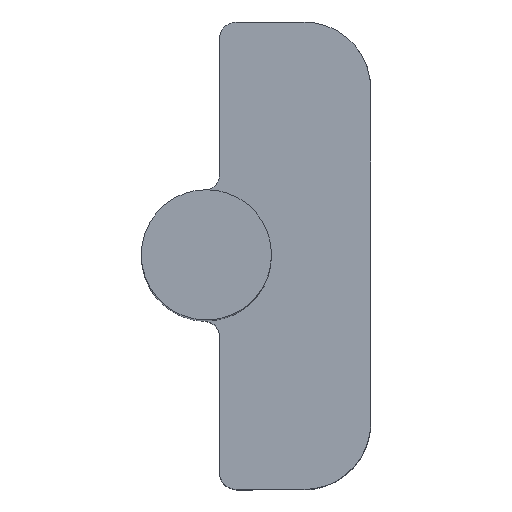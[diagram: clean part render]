
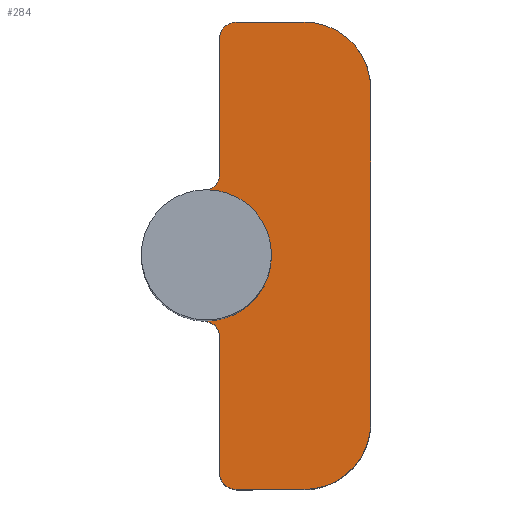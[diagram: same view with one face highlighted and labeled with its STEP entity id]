
A CAD part, top view. The second image highlights one B-rep face of the part: STEP entity #284.
In plain terms, the highlighted planar face has unit normal (0, 0, 1).
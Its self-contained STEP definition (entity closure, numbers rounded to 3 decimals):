
#15=CIRCLE('',#307,2.);
#21=CIRCLE('',#315,0.5);
#22=CIRCLE('',#318,0.5);
#24=CIRCLE('',#321,1.95);
#25=CIRCLE('',#322,1.95);
#26=CIRCLE('',#324,0.5);
#27=CIRCLE('',#327,0.5);
#28=CIRCLE('',#330,2.);
#47=FACE_OUTER_BOUND('',#63,.T.);
#63=EDGE_LOOP('',(#238,#239,#240,#241,#242,#243,#244,#245,#246,#247,#248,
#249,#250));
#79=LINE('',#468,#103);
#86=LINE('',#491,#110);
#88=LINE('',#497,#112);
#89=LINE('',#501,#113);
#90=LINE('',#502,#114);
#103=VECTOR('',#376,10.);
#110=VECTOR('',#401,10.);
#112=VECTOR('',#409,10.);
#113=VECTOR('',#414,10.);
#114=VECTOR('',#415,10.);
#122=VERTEX_POINT('',#436);
#123=VERTEX_POINT('',#438);
#132=VERTEX_POINT('',#460);
#133=VERTEX_POINT('',#461);
#134=VERTEX_POINT('',#466);
#135=VERTEX_POINT('',#470);
#136=VERTEX_POINT('',#471);
#138=VERTEX_POINT('',#478);
#139=VERTEX_POINT('',#480);
#140=VERTEX_POINT('',#485);
#141=VERTEX_POINT('',#486);
#142=VERTEX_POINT('',#493);
#143=VERTEX_POINT('',#499);
#149=EDGE_CURVE('',#122,#123,#15,.T.);
#160=EDGE_CURVE('',#132,#133,#21,.T.);
#164=EDGE_CURVE('',#134,#132,#79,.T.);
#165=EDGE_CURVE('',#135,#136,#22,.T.);
#170=EDGE_CURVE('',#139,#138,#24,.T.);
#172=EDGE_CURVE('',#138,#136,#25,.T.);
#173=EDGE_CURVE('',#140,#141,#26,.T.);
#176=EDGE_CURVE('',#141,#122,#86,.F.);
#177=EDGE_CURVE('',#139,#142,#27,.T.);
#179=EDGE_CURVE('',#140,#142,#88,.F.);
#180=EDGE_CURVE('',#143,#134,#28,.T.);
#181=EDGE_CURVE('',#123,#143,#89,.T.);
#182=EDGE_CURVE('',#135,#133,#90,.F.);
#238=ORIENTED_EDGE('',*,*,#160,.F.);
#239=ORIENTED_EDGE('',*,*,#164,.F.);
#240=ORIENTED_EDGE('',*,*,#180,.F.);
#241=ORIENTED_EDGE('',*,*,#181,.F.);
#242=ORIENTED_EDGE('',*,*,#149,.F.);
#243=ORIENTED_EDGE('',*,*,#176,.F.);
#244=ORIENTED_EDGE('',*,*,#173,.F.);
#245=ORIENTED_EDGE('',*,*,#179,.T.);
#246=ORIENTED_EDGE('',*,*,#177,.F.);
#247=ORIENTED_EDGE('',*,*,#170,.T.);
#248=ORIENTED_EDGE('',*,*,#172,.T.);
#249=ORIENTED_EDGE('',*,*,#165,.F.);
#250=ORIENTED_EDGE('',*,*,#182,.T.);
#269=PLANE('',#329);
#284=ADVANCED_FACE('',(#47),#269,.F.);
#307=AXIS2_PLACEMENT_3D('',#439,#348,#349);
#315=AXIS2_PLACEMENT_3D('',#462,#369,#370);
#318=AXIS2_PLACEMENT_3D('',#472,#379,#380);
#321=AXIS2_PLACEMENT_3D('',#481,#388,#389);
#322=AXIS2_PLACEMENT_3D('',#483,#391,#392);
#324=AXIS2_PLACEMENT_3D('',#487,#395,#396);
#327=AXIS2_PLACEMENT_3D('',#494,#404,#405);
#329=AXIS2_PLACEMENT_3D('',#498,#410,#411);
#330=AXIS2_PLACEMENT_3D('',#500,#412,#413);
#348=DIRECTION('center_axis',(0.,0.,
-1.));
#349=DIRECTION('ref_axis',(0.707,0.707,0.));
#369=DIRECTION('center_axis',(0.,0.,
-1.));
#370=DIRECTION('ref_axis',(-0.707,-0.707,0.));
#376=DIRECTION('',(-1.,0.,0.));
#379=DIRECTION('center_axis',(0.,0.,
1.));
#380=DIRECTION('ref_axis',(0.721,0.693,0.));
#388=DIRECTION('center_axis',(0.,0.,
-1.));
#389=DIRECTION('ref_axis',(-1.,0.,0.));
#391=DIRECTION('center_axis',(0.,0.,
-1.));
#392=DIRECTION('ref_axis',(-1.,0.,0.));
#395=DIRECTION('center_axis',(0.,0.,
-1.));
#396=DIRECTION('ref_axis',(-0.707,0.707,0.));
#401=DIRECTION('',(-1.,0.,0.));
#404=DIRECTION('center_axis',(0.,0.,
1.));
#405=DIRECTION('ref_axis',(0.721,-0.693,0.));
#409=DIRECTION('',(0.,1.,0.));
#410=DIRECTION('center_axis',(0.,0.,
-1.));
#411=DIRECTION('ref_axis',(0.,1.,0.));
#412=DIRECTION('center_axis',(0.,0.,
-1.));
#413=DIRECTION('ref_axis',(0.707,-0.707,0.));
#414=DIRECTION('',(0.,-1.,0.));
#415=DIRECTION('',(0.,1.,0.));
#436=CARTESIAN_POINT('',(2.922,7.,32.8));
#438=CARTESIAN_POINT('',(4.922,5.,32.8));
#439=CARTESIAN_POINT('Origin',(2.922,5.,32.8));
#460=CARTESIAN_POINT('',(0.9,-7.,32.8));
#461=CARTESIAN_POINT('',(0.4,-6.5,32.8));
#462=CARTESIAN_POINT('Origin',(0.9,-6.5,32.8));
#466=CARTESIAN_POINT('',(2.922,-7.,32.8));
#468=CARTESIAN_POINT('',(2.5,-7.,32.8));
#470=CARTESIAN_POINT('',(0.4,-2.448,32.8));
#471=CARTESIAN_POINT('',(-0.08,-1.948,32.8));
#472=CARTESIAN_POINT('Origin',(-0.1,-2.448,32.8));
#478=CARTESIAN_POINT('',(1.95,0.,32.8));
#480=CARTESIAN_POINT('',(-0.08,1.948,32.8));
#481=CARTESIAN_POINT('Origin',(0.,0.,
32.8));
#483=CARTESIAN_POINT('Origin',(0.,0.,
32.8));
#485=CARTESIAN_POINT('',(0.4,6.5,32.8));
#486=CARTESIAN_POINT('',(0.9,7.,32.8));
#487=CARTESIAN_POINT('Origin',(0.9,6.5,32.8));
#491=CARTESIAN_POINT('',(2.5,7.,32.8));
#493=CARTESIAN_POINT('',(0.4,2.448,32.8));
#494=CARTESIAN_POINT('Origin',(-0.1,2.448,32.8));
#497=CARTESIAN_POINT('',(0.4,3.45,32.8));
#498=CARTESIAN_POINT('Origin',(2.5,3.45,32.8));
#499=CARTESIAN_POINT('',(4.922,-5.,32.8));
#500=CARTESIAN_POINT('Origin',(2.922,-5.,32.8));
#501=CARTESIAN_POINT('',(4.922,3.45,32.8));
#502=CARTESIAN_POINT('',(0.4,3.45,32.8));
